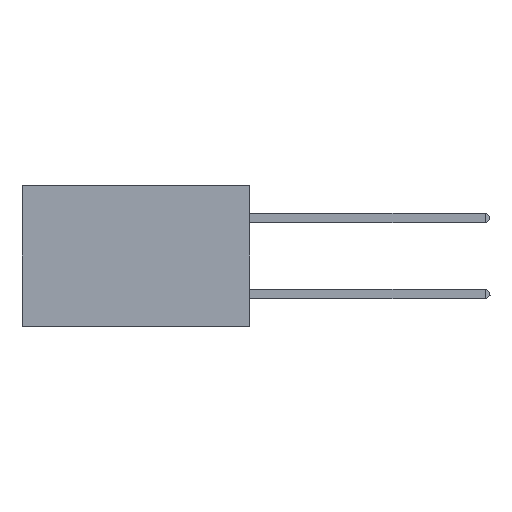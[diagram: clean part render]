
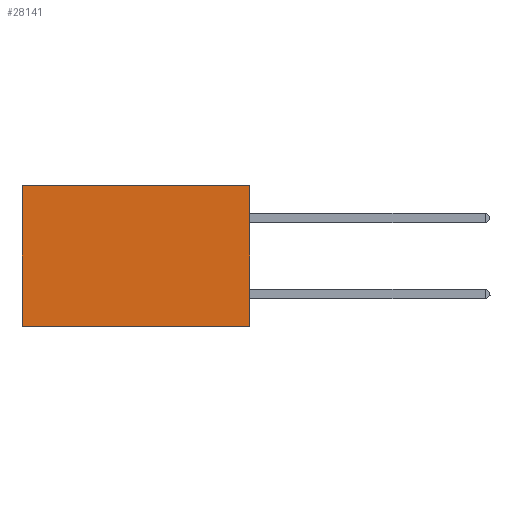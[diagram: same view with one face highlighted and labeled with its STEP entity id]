
A CAD part, left-side view. The second image highlights one B-rep face of the part: STEP entity #28141.
In plain terms, the highlighted planar face has unit normal (-1, 0, 0).
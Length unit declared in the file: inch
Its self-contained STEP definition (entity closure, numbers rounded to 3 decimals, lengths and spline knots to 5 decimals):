
#1622 = CARTESIAN_POINT ( 'NONE',  ( 0.2875, 0., -0.37 ) ) ;
#1740 = CARTESIAN_POINT ( 'NONE',  ( 0.2875, 0.6, 0. ) ) ;
#2285 = VECTOR ( 'NONE', #20714, 39.37008 ) ;
#4169 = PLANE ( 'NONE',  #10907 ) ;
#5857 = LINE ( 'NONE', #6252, #21011 ) ;
#6252 = CARTESIAN_POINT ( 'NONE',  ( 0.2875, 0., 0. ) ) ;
#9310 = VECTOR ( 'NONE', #37496, 39.37008 ) ;
#9678 = CARTESIAN_POINT ( 'NONE',  ( 0.2875, 0.6, -0.37 ) ) ;
#10368 = LINE ( 'NONE', #37483, #32602 ) ;
#10907 = AXIS2_PLACEMENT_3D ( 'NONE', #13576, #34850, #30327 ) ;
#11616 = ORIENTED_EDGE ( 'NONE', *, *, #11642, .T. ) ;
#11642 = EDGE_CURVE ( 'NONE', #33059, #30912, #12878, .T. ) ;
#12793 = EDGE_CURVE ( 'NONE', #16396, #30912, #22483, .T. ) ;
#12878 = LINE ( 'NONE', #36616, #2285 ) ;
#13576 = CARTESIAN_POINT ( 'NONE',  ( 0.2875, 0., 0. ) ) ;
#14025 = ORIENTED_EDGE ( 'NONE', *, *, #28334, .F. ) ;
#16138 = DIRECTION ( 'NONE',  ( 0., 1., 0. ) ) ;
#16396 = VERTEX_POINT ( 'NONE', #31541 ) ;
#17770 = CARTESIAN_POINT ( 'NONE',  ( 0.2875, 0., 0. ) ) ;
#18166 = DIRECTION ( 'NONE',  ( 0., 0., -1. ) ) ;
#19866 = VERTEX_POINT ( 'NONE', #17770 ) ;
#20265 = EDGE_LOOP ( 'NONE', ( #11616, #32707, #14025, #40469 ) ) ;
#20714 = DIRECTION ( 'NONE',  ( 0., 0., -1. ) ) ;
#21011 = VECTOR ( 'NONE', #16138, 39.37008 ) ;
#22483 = LINE ( 'NONE', #1622, #9310 ) ;
#28141 = ADVANCED_FACE ( 'NONE', ( #32104 ), #4169, .F. ) ;
#28334 = EDGE_CURVE ( 'NONE', #19866, #16396, #10368, .T. ) ;
#30327 = DIRECTION ( 'NONE',  ( 0., 0., -1. ) ) ;
#30912 = VERTEX_POINT ( 'NONE', #9678 ) ;
#31541 = CARTESIAN_POINT ( 'NONE',  ( 0.2875, 0., -0.37 ) ) ;
#32104 = FACE_OUTER_BOUND ( 'NONE', #20265, .T. ) ;
#32602 = VECTOR ( 'NONE', #18166, 39.37008 ) ;
#32707 = ORIENTED_EDGE ( 'NONE', *, *, #12793, .F. ) ;
#33059 = VERTEX_POINT ( 'NONE', #1740 ) ;
#34850 = DIRECTION ( 'NONE',  ( 1., 0., 0. ) ) ;
#35182 = EDGE_CURVE ( 'NONE', #19866, #33059, #5857, .T. ) ;
#36616 = CARTESIAN_POINT ( 'NONE',  ( 0.2875, 0.6, 0. ) ) ;
#37483 = CARTESIAN_POINT ( 'NONE',  ( 0.2875, 0., 0. ) ) ;
#37496 = DIRECTION ( 'NONE',  ( 0., 1., 0. ) ) ;
#40469 = ORIENTED_EDGE ( 'NONE', *, *, #35182, .T. ) ;
